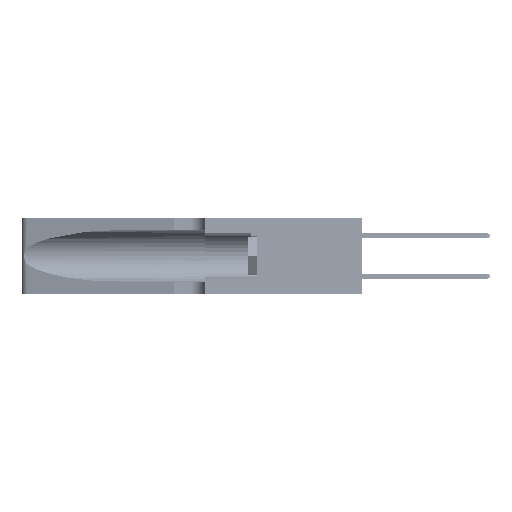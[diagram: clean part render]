
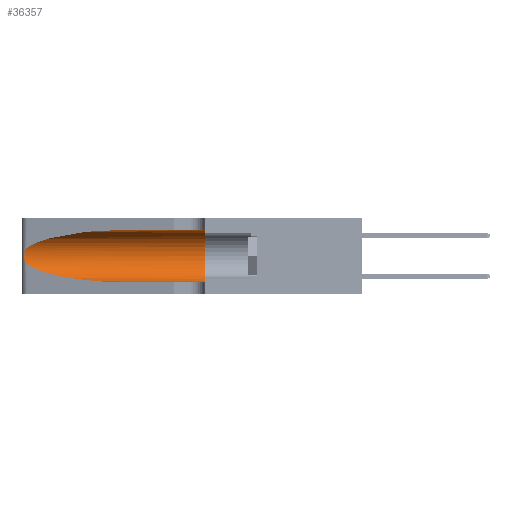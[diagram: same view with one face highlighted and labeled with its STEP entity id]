
A CAD part, left-side view. The second image highlights one B-rep face of the part: STEP entity #36357.
In plain terms, the highlighted cylindrical face has radius 3.308 mm (diameter 6.617 mm), a partial arc.
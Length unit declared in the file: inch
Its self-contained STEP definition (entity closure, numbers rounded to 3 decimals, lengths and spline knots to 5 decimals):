
#431 = EDGE_LOOP ( 'NONE', ( #29881, #12028, #6365, #16048, #2909, #8687 ) ) ;
#2909 = ORIENTED_EDGE ( 'NONE', *, *, #15447, .F. ) ;
#3500 = CARTESIAN_POINT ( 'NONE',  ( 0.26018, 1.23835, 0.19895 ) ) ;
#3668 = CARTESIAN_POINT ( 'NONE',  ( 0.26075, 1.23896, 0.178 ) ) ;
#4576 = VERTEX_POINT ( 'NONE', #33528 ) ;
#5559 = EDGE_CURVE ( 'NONE', #25756, #34044, #37668, .T. ) ;
#6365 = ORIENTED_EDGE ( 'NONE', *, *, #5559, .T. ) ;
#6614 = CARTESIAN_POINT ( 'NONE',  ( 0.18966, 0.96281, 0.05475 ) ) ;
#8687 = ORIENTED_EDGE ( 'NONE', *, *, #34003, .F. ) ;
#10746 = DIRECTION ( 'NONE',  ( 0., -1., 0. ) ) ;
#10965 =( BOUNDED_CURVE ( )  B_SPLINE_CURVE ( 3, ( #11600, #26827, #37879, #11774 ),
 .UNSPECIFIED., .F., .T. ) 
 B_SPLINE_CURVE_WITH_KNOTS ( ( 4, 4 ),
 ( 1.5708, 2.84003 ),
 .UNSPECIFIED. ) 
 CURVE ( )  GEOMETRIC_REPRESENTATION_ITEM ( )  RATIONAL_B_SPLINE_CURVE ( ( 1., 0.87, 0.87, 1. ) ) 
 REPRESENTATION_ITEM ( '' )  );
#11039 = CARTESIAN_POINT ( 'NONE',  ( 0.1305, 1.61858, 0.185 ) ) ;
#11047 = CARTESIAN_POINT ( 'NONE',  ( 0.25854, 1.2359, 0.20912 ) ) ;
#11221 = CARTESIAN_POINT ( 'NONE',  ( 0.26017, 1.23833, 0.17102 ) ) ;
#11600 = CARTESIAN_POINT ( 'NONE',  ( 0.1305, 0.72297, 0.31525 ) ) ;
#11774 = CARTESIAN_POINT ( 'NONE',  ( 0.25487, 1.22718, 0.22369 ) ) ;
#12028 = ORIENTED_EDGE ( 'NONE', *, *, #38400, .T. ) ;
#13887 = CARTESIAN_POINT ( 'NONE',  ( 0.25487, 1.22718, 0.14631 ) ) ;
#15257 = CARTESIAN_POINT ( 'NONE',  ( 0.25487, 1.22718, 0.14631 ) ) ;
#15447 = EDGE_CURVE ( 'NONE', #49280, #4576, #36380, .T. ) ;
#15736 = VECTOR ( 'NONE', #10746, 39.37008 ) ;
#16048 = ORIENTED_EDGE ( 'NONE', *, *, #25253, .T. ) ;
#17981 = CARTESIAN_POINT ( 'NONE',  ( 0.1305, 0.72297, 0.31525 ) ) ;
#18183 = CARTESIAN_POINT ( 'NONE',  ( 0.1305, 1.61858, 0.05475 ) ) ;
#21925 = CARTESIAN_POINT ( 'NONE',  ( 0.2373, 1.15595, 0.08982 ) ) ;
#22476 = CARTESIAN_POINT ( 'NONE',  ( 0.25787, 1.23484, 0.2124 ) ) ;
#22535 = DIRECTION ( 'NONE',  ( 0., 0., 1. ) ) ;
#22962 = CARTESIAN_POINT ( 'NONE',  ( 0.25856, 1.23593, 0.16098 ) ) ;
#23149 = EDGE_CURVE ( 'NONE', #33949, #38008, #10965, .T. ) ;
#25253 = EDGE_CURVE ( 'NONE', #34044, #4576, #40720, .T. ) ;
#25756 = VERTEX_POINT ( 'NONE', #32810 ) ;
#25848 = DIRECTION ( 'NONE',  ( 0., 1., 0. ) ) ;
#26341 = AXIS2_PLACEMENT_3D ( 'NONE', #45439, #25848, #22535 ) ;
#26776 = CARTESIAN_POINT ( 'NONE',  ( 0.25487, 1.22718, 0.22369 ) ) ;
#26827 = CARTESIAN_POINT ( 'NONE',  ( 0.18966, 0.96281, 0.31525 ) ) ;
#28794 = CARTESIAN_POINT ( 'NONE',  ( 0.25487, 1.22718, 0.22369 ) ) ;
#29881 = ORIENTED_EDGE ( 'NONE', *, *, #23149, .T. ) ;
#32810 = CARTESIAN_POINT ( 'NONE',  ( 0.25487, 1.22718, 0.14631 ) ) ;
#33528 = CARTESIAN_POINT ( 'NONE',  ( 0.1305, 0.35, 0.05475 ) ) ;
#33642 = CARTESIAN_POINT ( 'NONE',  ( 0.1305, 1.61858, 0.31525 ) ) ;
#33936 = DIRECTION ( 'NONE',  ( 0., 0., -1. ) ) ;
#33949 = VERTEX_POINT ( 'NONE', #17981 ) ;
#33950 = CARTESIAN_POINT ( 'NONE',  ( 0.25639, 1.23184, 0.21858 ) ) ;
#34003 = EDGE_CURVE ( 'NONE', #33949, #49280, #45641, .T. ) ;
#34044 = VERTEX_POINT ( 'NONE', #48578 ) ;
#34116 = CARTESIAN_POINT ( 'NONE',  ( 0.26075, 1.23896, 0.19203 ) ) ;
#34860 = CYLINDRICAL_SURFACE ( 'NONE', #48737, 0.13025 ) ;
#35304 = VECTOR ( 'NONE', #48774, 39.37008 ) ;
#36357 = ADVANCED_FACE ( 'NONE', ( #49250 ), #34860, .F. ) ;
#36380 = CIRCLE ( 'NONE', #26341, 0.13025 ) ;
#37668 =( BOUNDED_CURVE ( )  B_SPLINE_CURVE ( 3, ( #13887, #21925, #6614, #48503 ),
 .UNSPECIFIED., .F., .F. ) 
 B_SPLINE_CURVE_WITH_KNOTS ( ( 4, 4 ),
 ( 3.44316, 4.71239 ),
 .UNSPECIFIED. ) 
 CURVE ( )  GEOMETRIC_REPRESENTATION_ITEM ( )  RATIONAL_B_SPLINE_CURVE ( ( 1., 0.87, 0.87, 1. ) ) 
 REPRESENTATION_ITEM ( '' )  );
#37879 = CARTESIAN_POINT ( 'NONE',  ( 0.2373, 1.15595, 0.28018 ) ) ;
#37986 = CARTESIAN_POINT ( 'NONE',  ( 0.25789, 1.23486, 0.15765 ) ) ;
#38008 = VERTEX_POINT ( 'NONE', #28794 ) ;
#38157 = CARTESIAN_POINT ( 'NONE',  ( 0.25639, 1.23186, 0.15144 ) ) ;
#38400 = EDGE_CURVE ( 'NONE', #38008, #25756, #41982, .T. ) ;
#40720 = LINE ( 'NONE', #18183, #35304 ) ;
#41860 = CARTESIAN_POINT ( 'NONE',  ( 0.25555, 1.22993, 0.14849 ) ) ;
#41982 = B_SPLINE_CURVE_WITH_KNOTS ( 'NONE', 3,
 ( #26776, #45860, #33950, #22476, #11047, #3500, #34116, #3668, #11221, #22962, #37986, #38157, #41860, #15257 ),
 .UNSPECIFIED., .F., .F.,
 ( 4, 2, 2, 2, 2, 2, 4 ),
 ( 0., 0.00027, 0.00053, 0.00107, 0.0016, 0.00187, 0.00214 ),
 .UNSPECIFIED. ) ;
#45439 = CARTESIAN_POINT ( 'NONE',  ( 0.1305, 0.35, 0.185 ) ) ;
#45641 = LINE ( 'NONE', #33642, #15736 ) ;
#45860 = CARTESIAN_POINT ( 'NONE',  ( 0.25555, 1.22994, 0.2215 ) ) ;
#47473 = CARTESIAN_POINT ( 'NONE',  ( 0.1305, 0.35, 0.31525 ) ) ;
#48503 = CARTESIAN_POINT ( 'NONE',  ( 0.1305, 0.72297, 0.05475 ) ) ;
#48578 = CARTESIAN_POINT ( 'NONE',  ( 0.1305, 0.72297, 0.05475 ) ) ;
#48737 = AXIS2_PLACEMENT_3D ( 'NONE', #11039, #49035, #33936 ) ;
#48774 = DIRECTION ( 'NONE',  ( 0., -1., 0. ) ) ;
#49035 = DIRECTION ( 'NONE',  ( 0., -1., 0. ) ) ;
#49250 = FACE_OUTER_BOUND ( 'NONE', #431, .T. ) ;
#49280 = VERTEX_POINT ( 'NONE', #47473 ) ;
